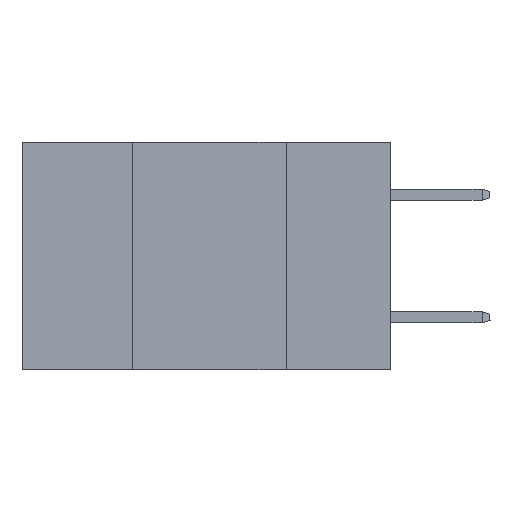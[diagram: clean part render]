
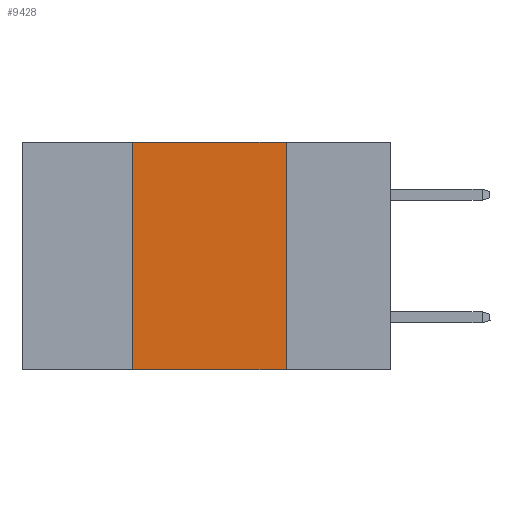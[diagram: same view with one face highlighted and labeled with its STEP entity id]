
A CAD part, left-side view. The second image highlights one B-rep face of the part: STEP entity #9428.
In plain terms, the highlighted planar face has unit normal (-1, 0, 0).
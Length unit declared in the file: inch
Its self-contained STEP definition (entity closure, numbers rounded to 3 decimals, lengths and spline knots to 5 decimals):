
#84 = LINE ( 'NONE', #9144, #4823 ) ;
#592 = PLANE ( 'NONE',  #8888 ) ;
#766 = LINE ( 'NONE', #4876, #3344 ) ;
#964 = CARTESIAN_POINT ( 'NONE',  ( 0., 0.6, 0. ) ) ;
#984 = EDGE_CURVE ( 'NONE', #8945, #10176, #8753, .T. ) ;
#1011 = LINE ( 'NONE', #7492, #7954 ) ;
#1296 = VECTOR ( 'NONE', #8149, 39.37008 ) ;
#1775 = CARTESIAN_POINT ( 'NONE',  ( 0., 0.42, -0.37 ) ) ;
#2725 = EDGE_CURVE ( 'NONE', #9579, #9721, #1011, .T. ) ;
#3344 = VECTOR ( 'NONE', #10145, 39.37008 ) ;
#3890 = EDGE_CURVE ( 'NONE', #9579, #8945, #84, .T. ) ;
#4429 = CARTESIAN_POINT ( 'NONE',  ( 0., 0.6, 0. ) ) ;
#4732 = CARTESIAN_POINT ( 'NONE',  ( 0., 0.17, -0.37 ) ) ;
#4823 = VECTOR ( 'NONE', #9109, 39.37008 ) ;
#4871 = ORIENTED_EDGE ( 'NONE', *, *, #2725, .T. ) ;
#4876 = CARTESIAN_POINT ( 'NONE',  ( 0., 0.17, 0. ) ) ;
#5292 = DIRECTION ( 'NONE',  ( 0., 0., -1. ) ) ;
#5830 = ORIENTED_EDGE ( 'NONE', *, *, #984, .F. ) ;
#6037 = CARTESIAN_POINT ( 'NONE',  ( 0., 0.17, 0. ) ) ;
#6301 = DIRECTION ( 'NONE',  ( 0., -1., 0. ) ) ;
#7492 = CARTESIAN_POINT ( 'NONE',  ( 0., 0.6, -0.37 ) ) ;
#7954 = VECTOR ( 'NONE', #6301, 39.37008 ) ;
#8149 = DIRECTION ( 'NONE',  ( 0., -1., 0. ) ) ;
#8292 = ORIENTED_EDGE ( 'NONE', *, *, #3890, .F. ) ;
#8753 = LINE ( 'NONE', #964, #1296 ) ;
#8806 = ORIENTED_EDGE ( 'NONE', *, *, #9810, .F. ) ;
#8888 = AXIS2_PLACEMENT_3D ( 'NONE', #4429, #10572, #5292 ) ;
#8945 = VERTEX_POINT ( 'NONE', #9218 ) ;
#9109 = DIRECTION ( 'NONE',  ( 0., 0., 1. ) ) ;
#9144 = CARTESIAN_POINT ( 'NONE',  ( 0., 0.42, 0. ) ) ;
#9218 = CARTESIAN_POINT ( 'NONE',  ( 0., 0.42, 0. ) ) ;
#9428 = ADVANCED_FACE ( 'NONE', ( #10651 ), #592, .F. ) ;
#9579 = VERTEX_POINT ( 'NONE', #1775 ) ;
#9721 = VERTEX_POINT ( 'NONE', #4732 ) ;
#9810 = EDGE_CURVE ( 'NONE', #10176, #9721, #766, .T. ) ;
#9964 = EDGE_LOOP ( 'NONE', ( #8806, #5830, #8292, #4871 ) ) ;
#10145 = DIRECTION ( 'NONE',  ( 0., 0., -1. ) ) ;
#10176 = VERTEX_POINT ( 'NONE', #6037 ) ;
#10572 = DIRECTION ( 'NONE',  ( 1., 0., 0. ) ) ;
#10651 = FACE_OUTER_BOUND ( 'NONE', #9964, .T. ) ;
